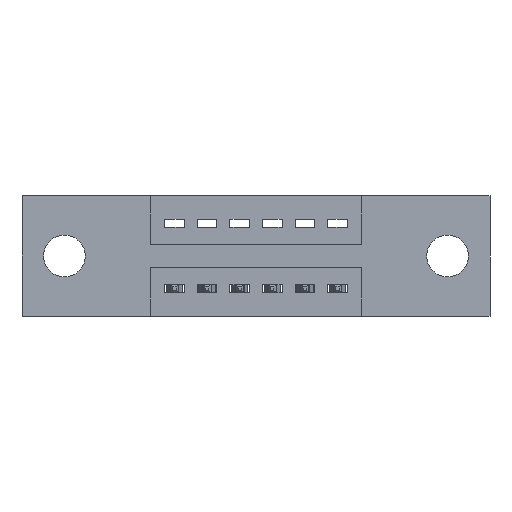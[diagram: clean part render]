
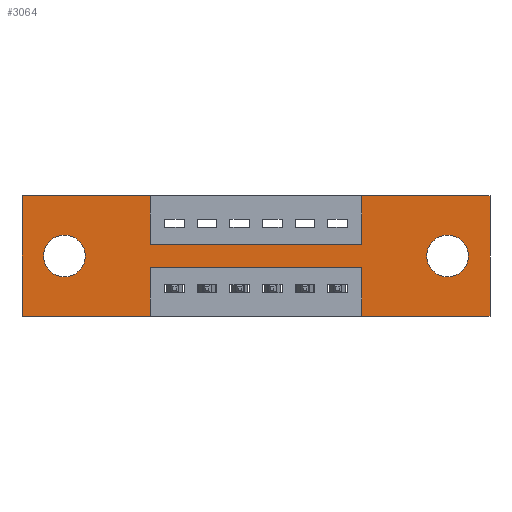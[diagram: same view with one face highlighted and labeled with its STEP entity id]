
A CAD part, front view. The second image highlights one B-rep face of the part: STEP entity #3064.
In plain terms, the highlighted planar face has unit normal (0, -1, 0).
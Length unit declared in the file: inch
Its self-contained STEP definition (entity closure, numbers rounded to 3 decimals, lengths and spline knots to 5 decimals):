
#36 = LINE ( 'NONE', #8619, #4221 ) ;
#372 = VERTEX_POINT ( 'NONE', #5355 ) ;
#390 = VERTEX_POINT ( 'NONE', #677 ) ;
#465 = ORIENTED_EDGE ( 'NONE', *, *, #3819, .F. ) ;
#596 = DIRECTION ( 'NONE',  ( 0., 0., 1. ) ) ;
#677 = CARTESIAN_POINT ( 'NONE',  ( 0.3925, 0., -0.22 ) ) ;
#837 = VECTOR ( 'NONE', #5877, 39.37008 ) ;
#880 = ORIENTED_EDGE ( 'NONE', *, *, #2143, .F. ) ;
#994 = EDGE_CURVE ( 'NONE', #7023, #9398, #2839, .T. ) ;
#1182 = CARTESIAN_POINT ( 'NONE',  ( 0., 0., 0. ) ) ;
#1270 = VERTEX_POINT ( 'NONE', #1983 ) ;
#1285 = FACE_BOUND ( 'NONE', #5652, .T. ) ;
#1291 = VERTEX_POINT ( 'NONE', #1182 ) ;
#1457 = VERTEX_POINT ( 'NONE', #3459 ) ;
#1649 = LINE ( 'NONE', #5894, #5446 ) ;
#1838 = VERTEX_POINT ( 'NONE', #9247 ) ;
#1877 = ORIENTED_EDGE ( 'NONE', *, *, #6954, .F. ) ;
#1983 = CARTESIAN_POINT ( 'NONE',  ( 0.3925, 0., 0. ) ) ;
#2015 = ORIENTED_EDGE ( 'NONE', *, *, #5118, .T. ) ;
#2063 = DIRECTION ( 'NONE',  ( -1., 0., 0. ) ) ;
#2091 = CARTESIAN_POINT ( 'NONE',  ( 0.3925, 0., -0.22 ) ) ;
#2143 = EDGE_CURVE ( 'NONE', #1838, #4981, #36, .T. ) ;
#2187 = VECTOR ( 'NONE', #3527, 39.37008 ) ;
#2204 = EDGE_CURVE ( 'NONE', #390, #1838, #6229, .T. ) ;
#2493 = VERTEX_POINT ( 'NONE', #6777 ) ;
#2532 = VERTEX_POINT ( 'NONE', #6467 ) ;
#2676 = DIRECTION ( 'NONE',  ( 0., 0., 1. ) ) ;
#2711 = EDGE_CURVE ( 'NONE', #8431, #2532, #4754, .T. ) ;
#2766 = DIRECTION ( 'NONE',  ( 0., 0., -1. ) ) ;
#2781 = DIRECTION ( 'NONE',  ( 0., 1., 0. ) ) ;
#2805 = CARTESIAN_POINT ( 'NONE',  ( 1.305, 0., -0.185 ) ) ;
#2839 = CIRCLE ( 'NONE', #5226, 0.064 ) ;
#2929 = ORIENTED_EDGE ( 'NONE', *, *, #4455, .T. ) ;
#3064 = ADVANCED_FACE ( 'NONE', ( #7339, #1285, #3784 ), #5035, .T. ) ;
#3269 = CIRCLE ( 'NONE', #8584, 0.064 ) ;
#3299 = CARTESIAN_POINT ( 'NONE',  ( 0.13, 0., -0.121 ) ) ;
#3459 = CARTESIAN_POINT ( 'NONE',  ( 1.435, 0., -0.37 ) ) ;
#3468 = DIRECTION ( 'NONE',  ( -1., 0., 0. ) ) ;
#3478 = CARTESIAN_POINT ( 'NONE',  ( 0., 0., 0. ) ) ;
#3491 = CARTESIAN_POINT ( 'NONE',  ( 0., 0., -0.37 ) ) ;
#3513 = DIRECTION ( 'NONE',  ( 1., 0., 0. ) ) ;
#3522 = VECTOR ( 'NONE', #2063, 39.37008 ) ;
#3527 = DIRECTION ( 'NONE',  ( 0., 0., -1. ) ) ;
#3576 = DIRECTION ( 'NONE',  ( 0., 0., 1. ) ) ;
#3604 = AXIS2_PLACEMENT_3D ( 'NONE', #4049, #3964, #4982 ) ;
#3608 = DIRECTION ( 'NONE',  ( 0., 0., 1. ) ) ;
#3618 = CARTESIAN_POINT ( 'NONE',  ( 1.0425, 0., -0.37 ) ) ;
#3619 = VECTOR ( 'NONE', #3576, 39.37008 ) ;
#3726 = CARTESIAN_POINT ( 'NONE',  ( 1.0425, 0., 0. ) ) ;
#3736 = CARTESIAN_POINT ( 'NONE',  ( 1.0425, 0., -0.15 ) ) ;
#3763 = VECTOR ( 'NONE', #3468, 39.37008 ) ;
#3784 = FACE_OUTER_BOUND ( 'NONE', #4346, .T. ) ;
#3819 = EDGE_CURVE ( 'NONE', #2493, #390, #7106, .T. ) ;
#3964 = DIRECTION ( 'NONE',  ( 0., -1., 0. ) ) ;
#4049 = CARTESIAN_POINT ( 'NONE',  ( 0., 0., -0.37 ) ) ;
#4050 = LINE ( 'NONE', #7604, #5656 ) ;
#4165 = VERTEX_POINT ( 'NONE', #7846 ) ;
#4218 = EDGE_CURVE ( 'NONE', #6458, #1457, #6799, .T. ) ;
#4221 = VECTOR ( 'NONE', #8670, 39.37008 ) ;
#4296 = DIRECTION ( 'NONE',  ( 1., 0., 0. ) ) ;
#4323 = ORIENTED_EDGE ( 'NONE', *, *, #2204, .F. ) ;
#4346 = EDGE_LOOP ( 'NONE', ( #4323, #465, #6537, #8648, #5414, #5630, #1877, #7543, #4435, #7956, #4654, #880 ) ) ;
#4389 = EDGE_CURVE ( 'NONE', #1457, #372, #7325, .T. ) ;
#4396 = VECTOR ( 'NONE', #3608, 39.37008 ) ;
#4435 = ORIENTED_EDGE ( 'NONE', *, *, #8267, .F. ) ;
#4455 = EDGE_CURVE ( 'NONE', #2532, #8431, #3269, .T. ) ;
#4606 = DIRECTION ( 'NONE',  ( 0., 1., 0. ) ) ;
#4654 = ORIENTED_EDGE ( 'NONE', *, *, #8940, .F. ) ;
#4736 = EDGE_CURVE ( 'NONE', #372, #2493, #7920, .T. ) ;
#4754 = CIRCLE ( 'NONE', #7093, 0.064 ) ;
#4791 = CARTESIAN_POINT ( 'NONE',  ( 0.13, 0., -0.185 ) ) ;
#4836 = VERTEX_POINT ( 'NONE', #6800 ) ;
#4981 = VERTEX_POINT ( 'NONE', #5956 ) ;
#4982 = DIRECTION ( 'NONE',  ( 0., 0., -1. ) ) ;
#5035 = PLANE ( 'NONE',  #3604 ) ;
#5118 = EDGE_CURVE ( 'NONE', #9398, #7023, #5266, .T. ) ;
#5226 = AXIS2_PLACEMENT_3D ( 'NONE', #4791, #7462, #596 ) ;
#5266 = CIRCLE ( 'NONE', #5676, 0.064 ) ;
#5306 = ORIENTED_EDGE ( 'NONE', *, *, #2711, .T. ) ;
#5355 = CARTESIAN_POINT ( 'NONE',  ( 1.0425, 0., -0.37 ) ) ;
#5414 = ORIENTED_EDGE ( 'NONE', *, *, #4218, .F. ) ;
#5446 = VECTOR ( 'NONE', #6540, 39.37008 ) ;
#5465 = LINE ( 'NONE', #3726, #3619 ) ;
#5630 = ORIENTED_EDGE ( 'NONE', *, *, #8320, .F. ) ;
#5633 = VECTOR ( 'NONE', #9170, 39.37008 ) ;
#5652 = EDGE_LOOP ( 'NONE', ( #5727, #2015 ) ) ;
#5656 = VECTOR ( 'NONE', #4296, 39.37008 ) ;
#5676 = AXIS2_PLACEMENT_3D ( 'NONE', #5879, #5858, #5849 ) ;
#5727 = ORIENTED_EDGE ( 'NONE', *, *, #994, .T. ) ;
#5790 = CARTESIAN_POINT ( 'NONE',  ( 1.435, 0., 0. ) ) ;
#5849 = DIRECTION ( 'NONE',  ( 0., 0., 1. ) ) ;
#5858 = DIRECTION ( 'NONE',  ( 0., 1., 0. ) ) ;
#5877 = DIRECTION ( 'NONE',  ( 0., 0., -1. ) ) ;
#5879 = CARTESIAN_POINT ( 'NONE',  ( 0.13, 0., -0.185 ) ) ;
#5894 = CARTESIAN_POINT ( 'NONE',  ( 0.3925, 0., -0.15 ) ) ;
#5956 = CARTESIAN_POINT ( 'NONE',  ( 0., 0., -0.37 ) ) ;
#6048 = LINE ( 'NONE', #6271, #2187 ) ;
#6135 = LINE ( 'NONE', #6852, #9152 ) ;
#6203 = CARTESIAN_POINT ( 'NONE',  ( 1.435, 0., 0. ) ) ;
#6229 = LINE ( 'NONE', #9180, #5633 ) ;
#6271 = CARTESIAN_POINT ( 'NONE',  ( 0.3925, 0., 0. ) ) ;
#6347 = EDGE_LOOP ( 'NONE', ( #2929, #5306 ) ) ;
#6458 = VERTEX_POINT ( 'NONE', #5790 ) ;
#6467 = CARTESIAN_POINT ( 'NONE',  ( 1.305, 0., -0.121 ) ) ;
#6537 = ORIENTED_EDGE ( 'NONE', *, *, #4736, .F. ) ;
#6540 = DIRECTION ( 'NONE',  ( 1., 0., 0. ) ) ;
#6572 = CARTESIAN_POINT ( 'NONE',  ( 1.305, 0., -0.185 ) ) ;
#6576 = VECTOR ( 'NONE', #3513, 39.37008 ) ;
#6589 = DIRECTION ( 'NONE',  ( 0., 0., -1. ) ) ;
#6777 = CARTESIAN_POINT ( 'NONE',  ( 1.0425, 0., -0.22 ) ) ;
#6799 = LINE ( 'NONE', #6203, #837 ) ;
#6800 = CARTESIAN_POINT ( 'NONE',  ( 0.3925, 0., -0.15 ) ) ;
#6852 = CARTESIAN_POINT ( 'NONE',  ( 0., 0., 0. ) ) ;
#6954 = EDGE_CURVE ( 'NONE', #7686, #4165, #5465, .T. ) ;
#7012 = EDGE_CURVE ( 'NONE', #1291, #1270, #8502, .T. ) ;
#7023 = VERTEX_POINT ( 'NONE', #3299 ) ;
#7056 = CARTESIAN_POINT ( 'NONE',  ( 1.305, 0., -0.249 ) ) ;
#7093 = AXIS2_PLACEMENT_3D ( 'NONE', #6572, #4606, #6589 ) ;
#7106 = LINE ( 'NONE', #2091, #3522 ) ;
#7325 = LINE ( 'NONE', #3491, #3763 ) ;
#7339 = FACE_BOUND ( 'NONE', #6347, .T. ) ;
#7462 = DIRECTION ( 'NONE',  ( 0., 1., 0. ) ) ;
#7543 = ORIENTED_EDGE ( 'NONE', *, *, #7830, .F. ) ;
#7604 = CARTESIAN_POINT ( 'NONE',  ( 0., 0., 0. ) ) ;
#7686 = VERTEX_POINT ( 'NONE', #3736 ) ;
#7830 = EDGE_CURVE ( 'NONE', #4836, #7686, #1649, .T. ) ;
#7846 = CARTESIAN_POINT ( 'NONE',  ( 1.0425, 0., 0. ) ) ;
#7920 = LINE ( 'NONE', #3618, #4396 ) ;
#7956 = ORIENTED_EDGE ( 'NONE', *, *, #7012, .F. ) ;
#8267 = EDGE_CURVE ( 'NONE', #1270, #4836, #6048, .T. ) ;
#8320 = EDGE_CURVE ( 'NONE', #4165, #6458, #4050, .T. ) ;
#8431 = VERTEX_POINT ( 'NONE', #7056 ) ;
#8502 = LINE ( 'NONE', #3478, #6576 ) ;
#8584 = AXIS2_PLACEMENT_3D ( 'NONE', #2805, #2781, #2766 ) ;
#8619 = CARTESIAN_POINT ( 'NONE',  ( 0., 0., -0.37 ) ) ;
#8621 = CARTESIAN_POINT ( 'NONE',  ( 0.13, 0., -0.249 ) ) ;
#8648 = ORIENTED_EDGE ( 'NONE', *, *, #4389, .F. ) ;
#8670 = DIRECTION ( 'NONE',  ( -1., 0., 0. ) ) ;
#8940 = EDGE_CURVE ( 'NONE', #4981, #1291, #6135, .T. ) ;
#9152 = VECTOR ( 'NONE', #2676, 39.37008 ) ;
#9170 = DIRECTION ( 'NONE',  ( 0., 0., -1. ) ) ;
#9180 = CARTESIAN_POINT ( 'NONE',  ( 0.3925, 0., -0.37 ) ) ;
#9247 = CARTESIAN_POINT ( 'NONE',  ( 0.3925, 0., -0.37 ) ) ;
#9398 = VERTEX_POINT ( 'NONE', #8621 ) ;
